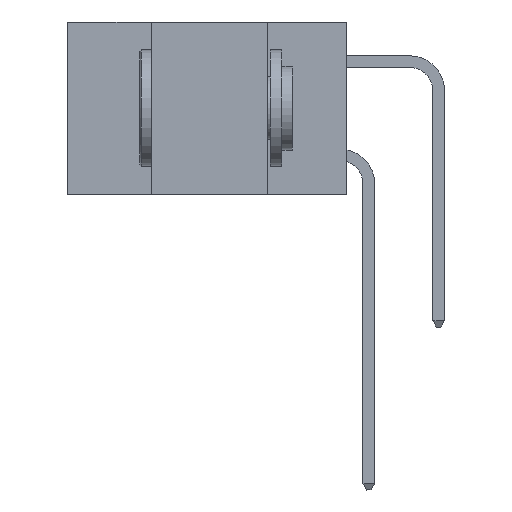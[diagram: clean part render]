
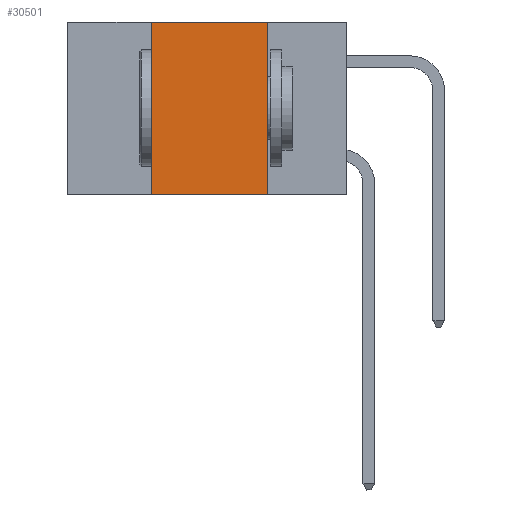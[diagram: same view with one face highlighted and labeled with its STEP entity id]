
A CAD part, left-side view. The second image highlights one B-rep face of the part: STEP entity #30501.
In plain terms, the highlighted planar face has unit normal (-1, 0, 0).
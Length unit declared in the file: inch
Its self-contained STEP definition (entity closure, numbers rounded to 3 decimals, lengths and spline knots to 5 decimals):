
#544 = EDGE_CURVE ( 'NONE', #14124, #1253, #11182, .T. ) ;
#1253 = VERTEX_POINT ( 'NONE', #19594 ) ;
#2944 = CARTESIAN_POINT ( 'NONE',  ( 0., 0.17, 0. ) ) ;
#4079 = LINE ( 'NONE', #23483, #24971 ) ;
#4391 = ORIENTED_EDGE ( 'NONE', *, *, #21690, .T. ) ;
#5637 = DIRECTION ( 'NONE',  ( 0., 0., -1. ) ) ;
#7218 = PLANE ( 'NONE',  #21359 ) ;
#7394 = CARTESIAN_POINT ( 'NONE',  ( 0., 0.42, -0.37 ) ) ;
#8264 = CARTESIAN_POINT ( 'NONE',  ( 0., 0.17, 0. ) ) ;
#11182 = LINE ( 'NONE', #8264, #15893 ) ;
#11335 = DIRECTION ( 'NONE',  ( 0., -1., 0. ) ) ;
#11860 = ORIENTED_EDGE ( 'NONE', *, *, #544, .F. ) ;
#12333 = FACE_OUTER_BOUND ( 'NONE', #31698, .T. ) ;
#12860 = CARTESIAN_POINT ( 'NONE',  ( 0., 0.6, 0. ) ) ;
#13869 = VERTEX_POINT ( 'NONE', #20189 ) ;
#14124 = VERTEX_POINT ( 'NONE', #2944 ) ;
#15893 = VECTOR ( 'NONE', #5637, 39.37008 ) ;
#17761 = LINE ( 'NONE', #31821, #31341 ) ;
#19594 = CARTESIAN_POINT ( 'NONE',  ( 0., 0.17, -0.37 ) ) ;
#19725 = CARTESIAN_POINT ( 'NONE',  ( 0., 0.6, -0.37 ) ) ;
#20189 = CARTESIAN_POINT ( 'NONE',  ( 0., 0.42, 0. ) ) ;
#20732 = EDGE_CURVE ( 'NONE', #32869, #13869, #4079, .T. ) ;
#21359 = AXIS2_PLACEMENT_3D ( 'NONE', #12860, #23643, #23294 ) ;
#21690 = EDGE_CURVE ( 'NONE', #32869, #1253, #22754, .T. ) ;
#22754 = LINE ( 'NONE', #19725, #32581 ) ;
#23294 = DIRECTION ( 'NONE',  ( 0., 0., -1. ) ) ;
#23483 = CARTESIAN_POINT ( 'NONE',  ( 0., 0.42, 0. ) ) ;
#23643 = DIRECTION ( 'NONE',  ( 1., 0., 0. ) ) ;
#24971 = VECTOR ( 'NONE', #26335, 39.37008 ) ;
#26335 = DIRECTION ( 'NONE',  ( 0., 0., 1. ) ) ;
#28500 = ORIENTED_EDGE ( 'NONE', *, *, #20732, .F. ) ;
#29163 = DIRECTION ( 'NONE',  ( 0., -1., 0. ) ) ;
#30501 = ADVANCED_FACE ( 'NONE', ( #12333 ), #7218, .F. ) ;
#31341 = VECTOR ( 'NONE', #29163, 39.37008 ) ;
#31698 = EDGE_LOOP ( 'NONE', ( #11860, #33494, #28500, #4391 ) ) ;
#31821 = CARTESIAN_POINT ( 'NONE',  ( 0., 0.6, 0. ) ) ;
#32581 = VECTOR ( 'NONE', #11335, 39.37008 ) ;
#32869 = VERTEX_POINT ( 'NONE', #7394 ) ;
#32933 = EDGE_CURVE ( 'NONE', #13869, #14124, #17761, .T. ) ;
#33494 = ORIENTED_EDGE ( 'NONE', *, *, #32933, .F. ) ;
